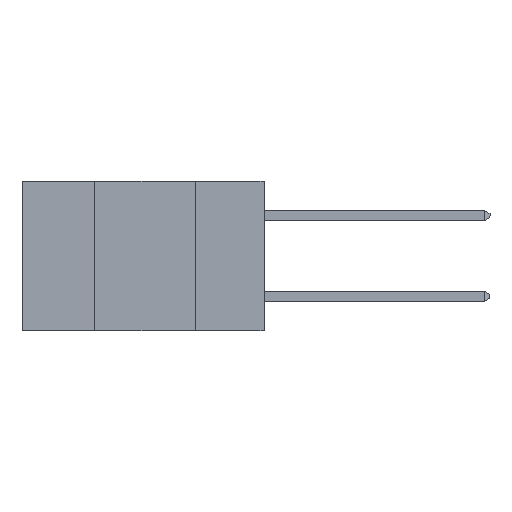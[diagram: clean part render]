
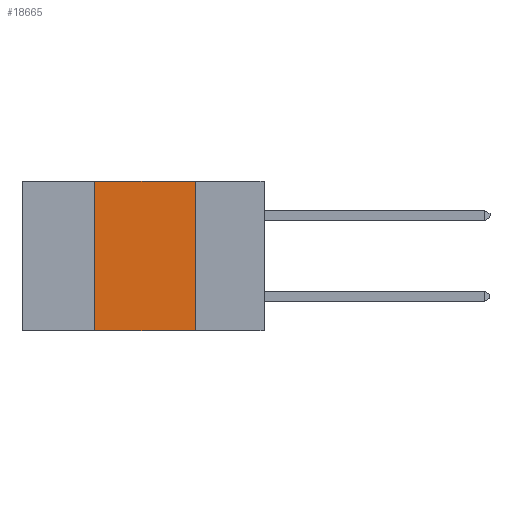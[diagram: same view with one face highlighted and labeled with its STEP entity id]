
A CAD part, left-side view. The second image highlights one B-rep face of the part: STEP entity #18665.
In plain terms, the highlighted planar face has unit normal (-1, 0, 0).
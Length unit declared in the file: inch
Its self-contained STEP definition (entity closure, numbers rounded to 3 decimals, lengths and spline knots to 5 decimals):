
#2072 = CARTESIAN_POINT ( 'NONE',  ( 0., 0.6, 0. ) ) ;
#2738 = EDGE_LOOP ( 'NONE', ( #21887, #23214, #7554, #21591 ) ) ;
#3782 = VECTOR ( 'NONE', #3902, 39.37008 ) ;
#3902 = DIRECTION ( 'NONE',  ( 0., -1., 0. ) ) ;
#4135 = VECTOR ( 'NONE', #10145, 39.37008 ) ;
#4248 = DIRECTION ( 'NONE',  ( 0., 0., -1. ) ) ;
#5226 = VERTEX_POINT ( 'NONE', #23088 ) ;
#5318 = CARTESIAN_POINT ( 'NONE',  ( 0., 0.17, 0. ) ) ;
#6493 = VECTOR ( 'NONE', #14591, 39.37008 ) ;
#6582 = EDGE_CURVE ( 'NONE', #5226, #13148, #21141, .T. ) ;
#7108 = VERTEX_POINT ( 'NONE', #24063 ) ;
#7554 = ORIENTED_EDGE ( 'NONE', *, *, #6582, .F. ) ;
#9464 = LINE ( 'NONE', #5318, #20118 ) ;
#10145 = DIRECTION ( 'NONE',  ( 0., 0., 1. ) ) ;
#10189 = CARTESIAN_POINT ( 'NONE',  ( 0., 0.42, 0. ) ) ;
#12769 = PLANE ( 'NONE',  #16135 ) ;
#12878 = LINE ( 'NONE', #23097, #6493 ) ;
#12904 = FACE_OUTER_BOUND ( 'NONE', #2738, .T. ) ;
#13081 = EDGE_CURVE ( 'NONE', #13148, #7108, #12878, .T. ) ;
#13148 = VERTEX_POINT ( 'NONE', #27400 ) ;
#13692 = EDGE_CURVE ( 'NONE', #5226, #18744, #20787, .T. ) ;
#14591 = DIRECTION ( 'NONE',  ( 0., -1., 0. ) ) ;
#16135 = AXIS2_PLACEMENT_3D ( 'NONE', #2072, #17030, #4248 ) ;
#17030 = DIRECTION ( 'NONE',  ( 1., 0., 0. ) ) ;
#18665 = ADVANCED_FACE ( 'NONE', ( #12904 ), #12769, .F. ) ;
#18744 = VERTEX_POINT ( 'NONE', #19405 ) ;
#18809 = CARTESIAN_POINT ( 'NONE',  ( 0., 0.6, -0.37 ) ) ;
#19405 = CARTESIAN_POINT ( 'NONE',  ( 0., 0.17, -0.37 ) ) ;
#19674 = EDGE_CURVE ( 'NONE', #7108, #18744, #9464, .T. ) ;
#20118 = VECTOR ( 'NONE', #22341, 39.37008 ) ;
#20787 = LINE ( 'NONE', #18809, #3782 ) ;
#21141 = LINE ( 'NONE', #10189, #4135 ) ;
#21591 = ORIENTED_EDGE ( 'NONE', *, *, #13692, .T. ) ;
#21887 = ORIENTED_EDGE ( 'NONE', *, *, #19674, .F. ) ;
#22341 = DIRECTION ( 'NONE',  ( 0., 0., -1. ) ) ;
#23088 = CARTESIAN_POINT ( 'NONE',  ( 0., 0.42, -0.37 ) ) ;
#23097 = CARTESIAN_POINT ( 'NONE',  ( 0., 0.6, 0. ) ) ;
#23214 = ORIENTED_EDGE ( 'NONE', *, *, #13081, .F. ) ;
#24063 = CARTESIAN_POINT ( 'NONE',  ( 0., 0.17, 0. ) ) ;
#27400 = CARTESIAN_POINT ( 'NONE',  ( 0., 0.42, 0. ) ) ;
